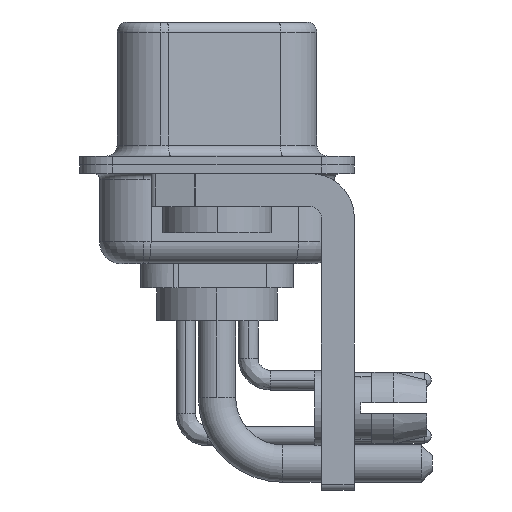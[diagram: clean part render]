
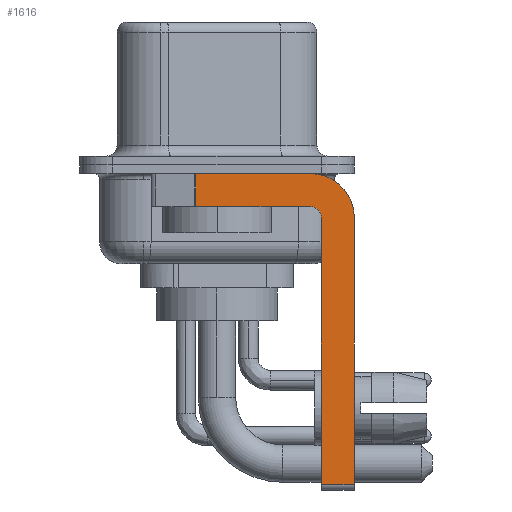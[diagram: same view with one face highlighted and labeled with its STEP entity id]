
A CAD part, left-side view. The second image highlights one B-rep face of the part: STEP entity #1616.
In plain terms, the highlighted planar face has unit normal (-1, 0, 0).
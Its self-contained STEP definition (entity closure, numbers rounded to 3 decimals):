
#387 = LINE ( 'NONE', #9421, #26474 ) ;
#669 = EDGE_CURVE ( 'NONE', #21353, #13918, #24544, .T. ) ;
#898 = CARTESIAN_POINT ( 'NONE',  ( -2.9, -6.25, -14.55 ) ) ;
#920 = ORIENTED_EDGE ( 'NONE', *, *, #20059, .F. ) ;
#931 = VERTEX_POINT ( 'NONE', #24223 ) ;
#1032 = LINE ( 'NONE', #26543, #6838 ) ;
#1616 = ADVANCED_FACE ( 'NONE', ( #5473 ), #14541, .F. ) ;
#1953 = CIRCLE ( 'NONE', #16161, 2. ) ;
#3411 = DIRECTION ( 'NONE',  ( 1., 0., 0. ) ) ;
#3640 = LINE ( 'NONE', #12691, #16997 ) ;
#3838 = DIRECTION ( 'NONE',  ( 0., 0., -1. ) ) ;
#4565 = EDGE_CURVE ( 'NONE', #5244, #22867, #22362, .T. ) ;
#4713 = ORIENTED_EDGE ( 'NONE', *, *, #16530, .F. ) ;
#5244 = VERTEX_POINT ( 'NONE', #17249 ) ;
#5473 = FACE_OUTER_BOUND ( 'NONE', #22707, .T. ) ;
#6583 = CARTESIAN_POINT ( 'NONE',  ( -2.9, -4.25, -0.4 ) ) ;
#6838 = VECTOR ( 'NONE', #19280, 1000. ) ;
#7621 = DIRECTION ( 'NONE',  ( 0., 0., -1. ) ) ;
#8039 = DIRECTION ( 'NONE',  ( 0., 0., 1. ) ) ;
#8126 = ORIENTED_EDGE ( 'NONE', *, *, #669, .F. ) ;
#8283 = CARTESIAN_POINT ( 'NONE',  ( -2.9, -4.25, -2.4 ) ) ;
#8884 = DIRECTION ( 'NONE',  ( -1., 0., 0. ) ) ;
#9421 = CARTESIAN_POINT ( 'NONE',  ( -2.9, -4.75, -14.8 ) ) ;
#10091 = VERTEX_POINT ( 'NONE', #26901 ) ;
#10099 = DIRECTION ( 'NONE',  ( 0., 1., 0. ) ) ;
#10567 = CARTESIAN_POINT ( 'NONE',  ( -2.9, -4.75, -2.4 ) ) ;
#10794 = ORIENTED_EDGE ( 'NONE', *, *, #20191, .T. ) ;
#10960 = DIRECTION ( 'NONE',  ( 1., 0., 0. ) ) ;
#11044 = CARTESIAN_POINT ( 'NONE',  ( -2.9, 3., -0.4 ) ) ;
#11084 = CARTESIAN_POINT ( 'NONE',  ( -2.9, -6.25, -2.4 ) ) ;
#12691 = CARTESIAN_POINT ( 'NONE',  ( -2.9, 0.978, -1.9 ) ) ;
#13448 = EDGE_CURVE ( 'NONE', #10091, #22867, #1032, .T. ) ;
#13480 = VERTEX_POINT ( 'NONE', #24306 ) ;
#13638 = CARTESIAN_POINT ( 'NONE',  ( -2.9, -4.25, -2.4 ) ) ;
#13918 = VERTEX_POINT ( 'NONE', #6583 ) ;
#14541 = PLANE ( 'NONE',  #14937 ) ;
#14937 = AXIS2_PLACEMENT_3D ( 'NONE', #18984, #3411, #23900 ) ;
#15082 = ORIENTED_EDGE ( 'NONE', *, *, #23027, .F. ) ;
#16161 = AXIS2_PLACEMENT_3D ( 'NONE', #8283, #10960, #3838 ) ;
#16530 = EDGE_CURVE ( 'NONE', #18689, #931, #22600, .T. ) ;
#16882 = ORIENTED_EDGE ( 'NONE', *, *, #4565, .F. ) ;
#16997 = VECTOR ( 'NONE', #7621, 1000. ) ;
#17249 = CARTESIAN_POINT ( 'NONE',  ( -2.9, -6.25, -2.4 ) ) ;
#17722 = DIRECTION ( 'NONE',  ( 0., -1., 0. ) ) ;
#18233 = ORIENTED_EDGE ( 'NONE', *, *, #19295, .F. ) ;
#18374 = VECTOR ( 'NONE', #10099, 1000. ) ;
#18689 = VERTEX_POINT ( 'NONE', #10567 ) ;
#18984 = CARTESIAN_POINT ( 'NONE',  ( -2.9, -4.25, -2.4 ) ) ;
#19280 = DIRECTION ( 'NONE',  ( 0., -1., 0. ) ) ;
#19295 = EDGE_CURVE ( 'NONE', #931, #13480, #24186, .T. ) ;
#19747 = AXIS2_PLACEMENT_3D ( 'NONE', #13638, #8884, #8039 ) ;
#20059 = EDGE_CURVE ( 'NONE', #10091, #18689, #387, .T. ) ;
#20191 = EDGE_CURVE ( 'NONE', #21353, #13480, #3640, .T. ) ;
#20414 = CARTESIAN_POINT ( 'NONE',  ( -2.9, 0.978, -0.4 ) ) ;
#21353 = VERTEX_POINT ( 'NONE', #20414 ) ;
#22362 = LINE ( 'NONE', #11084, #24333 ) ;
#22600 = CIRCLE ( 'NONE', #19747, 0.5 ) ;
#22707 = EDGE_LOOP ( 'NONE', ( #8126, #10794, #18233, #4713, #920, #25439, #16882, #15082 ) ) ;
#22867 = VERTEX_POINT ( 'NONE', #898 ) ;
#23027 = EDGE_CURVE ( 'NONE', #13918, #5244, #1953, .T. ) ;
#23098 = DIRECTION ( 'NONE',  ( 0., 0., 1. ) ) ;
#23900 = DIRECTION ( 'NONE',  ( 0., 0., -1. ) ) ;
#24186 = LINE ( 'NONE', #28224, #18374 ) ;
#24223 = CARTESIAN_POINT ( 'NONE',  ( -2.9, -4.25, -1.9 ) ) ;
#24306 = CARTESIAN_POINT ( 'NONE',  ( -2.9, 0.978, -1.9 ) ) ;
#24333 = VECTOR ( 'NONE', #26977, 1000. ) ;
#24544 = LINE ( 'NONE', #11044, #25781 ) ;
#25439 = ORIENTED_EDGE ( 'NONE', *, *, #13448, .T. ) ;
#25781 = VECTOR ( 'NONE', #17722, 1000. ) ;
#26474 = VECTOR ( 'NONE', #23098, 1000. ) ;
#26543 = CARTESIAN_POINT ( 'NONE',  ( -2.9, -4.25, -14.55 ) ) ;
#26901 = CARTESIAN_POINT ( 'NONE',  ( -2.9, -4.75, -14.55 ) ) ;
#26977 = DIRECTION ( 'NONE',  ( 0., 0., -1. ) ) ;
#28224 = CARTESIAN_POINT ( 'NONE',  ( -2.9, -4.25, -1.9 ) ) ;
